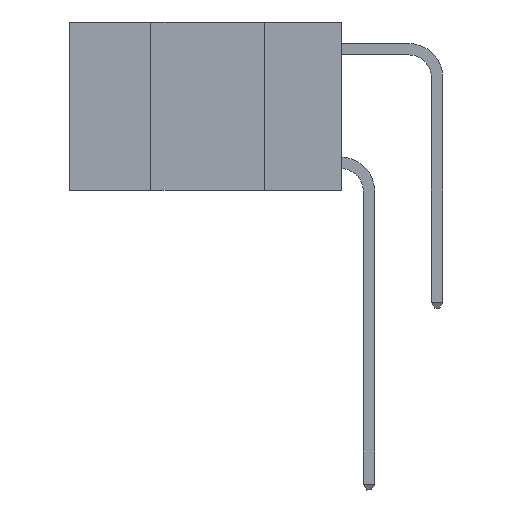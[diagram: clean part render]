
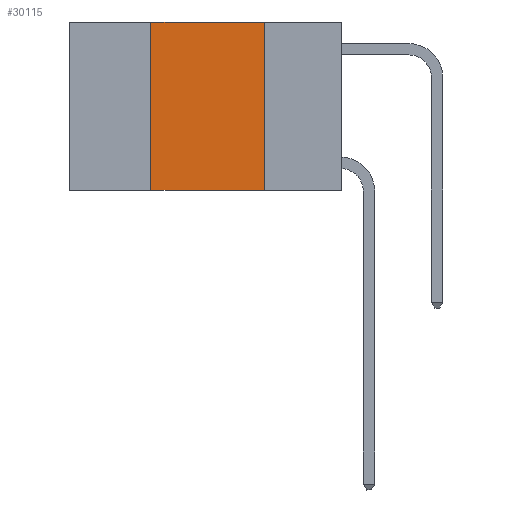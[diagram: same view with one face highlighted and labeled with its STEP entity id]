
A CAD part, left-side view. The second image highlights one B-rep face of the part: STEP entity #30115.
In plain terms, the highlighted planar face has unit normal (-1, 0, 0).
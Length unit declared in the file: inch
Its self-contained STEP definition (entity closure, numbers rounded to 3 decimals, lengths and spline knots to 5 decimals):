
#853 = CARTESIAN_POINT ( 'NONE',  ( 0., 0.17, 0. ) ) ;
#1497 = VERTEX_POINT ( 'NONE', #2895 ) ;
#2895 = CARTESIAN_POINT ( 'NONE',  ( 0., 0.17, 0. ) ) ;
#3053 = DIRECTION ( 'NONE',  ( 1., 0., 0. ) ) ;
#3215 = DIRECTION ( 'NONE',  ( 0., -1., 0. ) ) ;
#3251 = FACE_OUTER_BOUND ( 'NONE', #6679, .T. ) ;
#5149 = LINE ( 'NONE', #13475, #10715 ) ;
#6318 = DIRECTION ( 'NONE',  ( 0., 0., 1. ) ) ;
#6554 = ORIENTED_EDGE ( 'NONE', *, *, #10023, .F. ) ;
#6679 = EDGE_LOOP ( 'NONE', ( #13952, #6554, #27493, #18673 ) ) ;
#6991 = VERTEX_POINT ( 'NONE', #19194 ) ;
#10023 = EDGE_CURVE ( 'NONE', #19181, #1497, #26914, .T. ) ;
#10715 = VECTOR ( 'NONE', #6318, 39.37008 ) ;
#10823 = VERTEX_POINT ( 'NONE', #25201 ) ;
#12808 = LINE ( 'NONE', #853, #29370 ) ;
#13475 = CARTESIAN_POINT ( 'NONE',  ( 0., 0.42, 0. ) ) ;
#13952 = ORIENTED_EDGE ( 'NONE', *, *, #24229, .F. ) ;
#17222 = CARTESIAN_POINT ( 'NONE',  ( 0., 0.6, 0. ) ) ;
#17881 = EDGE_CURVE ( 'NONE', #10823, #19181, #5149, .T. ) ;
#18673 = ORIENTED_EDGE ( 'NONE', *, *, #30111, .T. ) ;
#19181 = VERTEX_POINT ( 'NONE', #23427 ) ;
#19194 = CARTESIAN_POINT ( 'NONE',  ( 0., 0.17, -0.37 ) ) ;
#19575 = DIRECTION ( 'NONE',  ( 0., 0., -1. ) ) ;
#19640 = CARTESIAN_POINT ( 'NONE',  ( 0., 0.6, 0. ) ) ;
#19753 = DIRECTION ( 'NONE',  ( 0., 0., -1. ) ) ;
#20678 = VECTOR ( 'NONE', #3215, 39.37008 ) ;
#21829 = AXIS2_PLACEMENT_3D ( 'NONE', #17222, #3053, #19575 ) ;
#23427 = CARTESIAN_POINT ( 'NONE',  ( 0., 0.42, 0. ) ) ;
#23613 = LINE ( 'NONE', #26495, #28355 ) ;
#24229 = EDGE_CURVE ( 'NONE', #1497, #6991, #12808, .T. ) ;
#24247 = DIRECTION ( 'NONE',  ( 0., -1., 0. ) ) ;
#25201 = CARTESIAN_POINT ( 'NONE',  ( 0., 0.42, -0.37 ) ) ;
#26495 = CARTESIAN_POINT ( 'NONE',  ( 0., 0.6, -0.37 ) ) ;
#26593 = PLANE ( 'NONE',  #21829 ) ;
#26914 = LINE ( 'NONE', #19640, #20678 ) ;
#27493 = ORIENTED_EDGE ( 'NONE', *, *, #17881, .F. ) ;
#28355 = VECTOR ( 'NONE', #24247, 39.37008 ) ;
#29370 = VECTOR ( 'NONE', #19753, 39.37008 ) ;
#30111 = EDGE_CURVE ( 'NONE', #10823, #6991, #23613, .T. ) ;
#30115 = ADVANCED_FACE ( 'NONE', ( #3251 ), #26593, .F. ) ;
